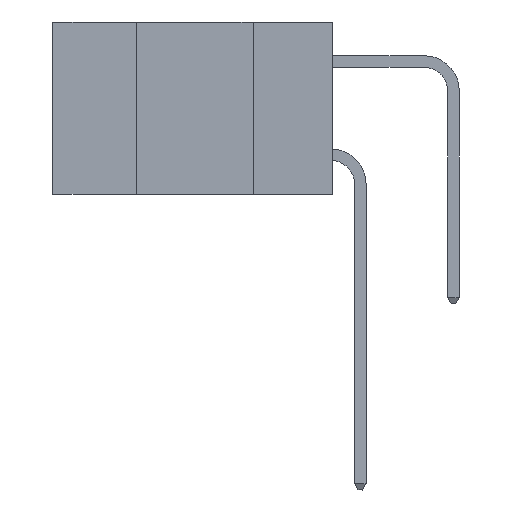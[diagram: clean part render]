
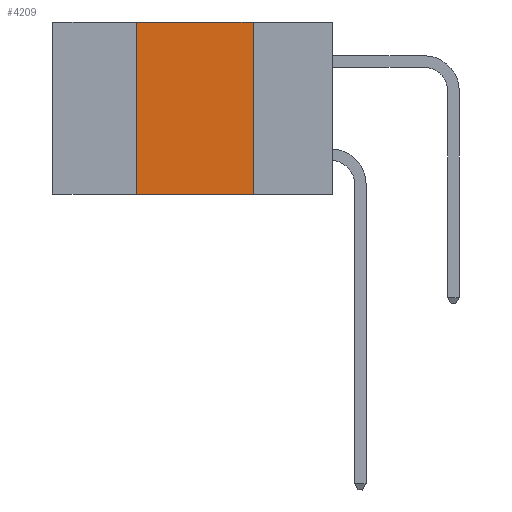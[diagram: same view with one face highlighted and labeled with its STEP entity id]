
A CAD part, left-side view. The second image highlights one B-rep face of the part: STEP entity #4209.
In plain terms, the highlighted planar face has unit normal (-1, 0, 0).
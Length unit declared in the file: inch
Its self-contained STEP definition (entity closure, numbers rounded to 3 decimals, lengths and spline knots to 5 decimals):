
#1381 = VECTOR ( 'NONE', #15454, 39.37008 ) ;
#2179 = CARTESIAN_POINT ( 'NONE',  ( 0., 0.17, 0. ) ) ;
#2397 = CARTESIAN_POINT ( 'NONE',  ( 0., 0.6, -0.37 ) ) ;
#3212 = VECTOR ( 'NONE', #25885, 39.37008 ) ;
#3564 = LINE ( 'NONE', #2397, #34335 ) ;
#3649 = VERTEX_POINT ( 'NONE', #19996 ) ;
#3917 = ORIENTED_EDGE ( 'NONE', *, *, #31419, .T. ) ;
#4209 = ADVANCED_FACE ( 'NONE', ( #17147 ), #14215, .F. ) ;
#5736 = CARTESIAN_POINT ( 'NONE',  ( 0., 0.42, 0. ) ) ;
#8745 = DIRECTION ( 'NONE',  ( 0., 0., 1. ) ) ;
#8853 = CARTESIAN_POINT ( 'NONE',  ( 0., 0.42, -0.37 ) ) ;
#10122 = LINE ( 'NONE', #28756, #1381 ) ;
#10242 = EDGE_CURVE ( 'NONE', #10991, #3649, #13164, .T. ) ;
#10928 = ORIENTED_EDGE ( 'NONE', *, *, #23036, .F. ) ;
#10991 = VERTEX_POINT ( 'NONE', #20893 ) ;
#11457 = DIRECTION ( 'NONE',  ( 0., 0., -1. ) ) ;
#11749 = VERTEX_POINT ( 'NONE', #25586 ) ;
#11863 = VECTOR ( 'NONE', #8745, 39.37008 ) ;
#12692 = LINE ( 'NONE', #5736, #11863 ) ;
#13164 = LINE ( 'NONE', #2179, #3212 ) ;
#14215 = PLANE ( 'NONE',  #24011 ) ;
#14974 = ORIENTED_EDGE ( 'NONE', *, *, #31565, .F. ) ;
#15454 = DIRECTION ( 'NONE',  ( 0., -1., 0. ) ) ;
#17147 = FACE_OUTER_BOUND ( 'NONE', #17703, .T. ) ;
#17703 = EDGE_LOOP ( 'NONE', ( #18768, #10928, #14974, #3917 ) ) ;
#18768 = ORIENTED_EDGE ( 'NONE', *, *, #10242, .F. ) ;
#19996 = CARTESIAN_POINT ( 'NONE',  ( 0., 0.17, -0.37 ) ) ;
#20893 = CARTESIAN_POINT ( 'NONE',  ( 0., 0.17, 0. ) ) ;
#21823 = CARTESIAN_POINT ( 'NONE',  ( 0., 0.6, 0. ) ) ;
#22747 = VERTEX_POINT ( 'NONE', #8853 ) ;
#23036 = EDGE_CURVE ( 'NONE', #11749, #10991, #10122, .T. ) ;
#23330 = DIRECTION ( 'NONE',  ( 0., -1., 0. ) ) ;
#24011 = AXIS2_PLACEMENT_3D ( 'NONE', #21823, #27176, #11457 ) ;
#25586 = CARTESIAN_POINT ( 'NONE',  ( 0., 0.42, 0. ) ) ;
#25885 = DIRECTION ( 'NONE',  ( 0., 0., -1. ) ) ;
#27176 = DIRECTION ( 'NONE',  ( 1., 0., 0. ) ) ;
#28756 = CARTESIAN_POINT ( 'NONE',  ( 0., 0.6, 0. ) ) ;
#31419 = EDGE_CURVE ( 'NONE', #22747, #3649, #3564, .T. ) ;
#31565 = EDGE_CURVE ( 'NONE', #22747, #11749, #12692, .T. ) ;
#34335 = VECTOR ( 'NONE', #23330, 39.37008 ) ;
